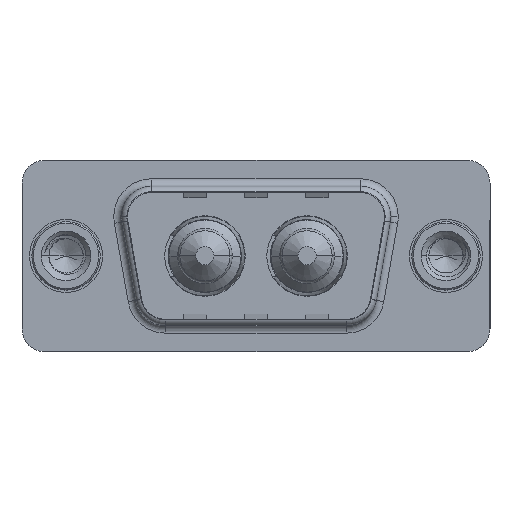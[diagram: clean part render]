
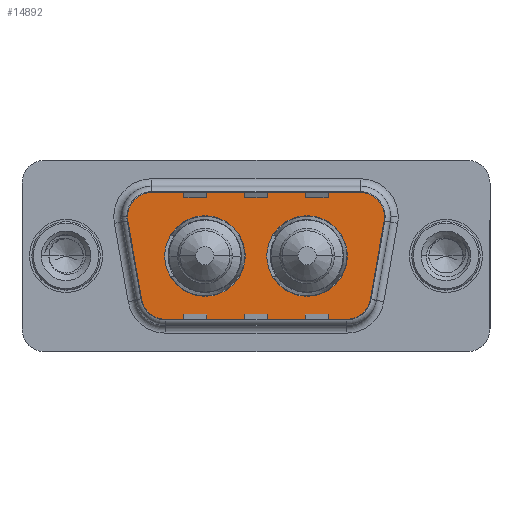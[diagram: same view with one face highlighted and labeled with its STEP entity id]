
A CAD part, top view. The second image highlights one B-rep face of the part: STEP entity #14892.
In plain terms, the highlighted planar face has unit normal (0, 0, 1).
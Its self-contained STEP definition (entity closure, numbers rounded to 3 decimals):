
#26 = CARTESIAN_POINT ( 'NONE',  ( 6.459, -4.9, 0. ) ) ;
#253 = ORIENTED_EDGE ( 'NONE', *, *, #2619, .T. ) ;
#300 = VERTEX_POINT ( 'NONE', #6458 ) ;
#446 = ORIENTED_EDGE ( 'NONE', *, *, #7942, .T. ) ;
#957 = LINE ( 'NONE', #13307, #3963 ) ;
#961 = CARTESIAN_POINT ( 'NONE',  ( 6.459, -2.9, 0. ) ) ;
#1237 = CARTESIAN_POINT ( 'NONE',  ( 15.86, 0., 0. ) ) ;
#1361 = CIRCLE ( 'NONE', #2441, 2. ) ;
#1375 = VERTEX_POINT ( 'NONE', #12462 ) ;
#1765 = ORIENTED_EDGE ( 'NONE', *, *, #13793, .F. ) ;
#1988 = VERTEX_POINT ( 'NONE', #5027 ) ;
#2060 = DIRECTION ( 'NONE',  ( -1., 0., 0. ) ) ;
#2064 = ORIENTED_EDGE ( 'NONE', *, *, #10052, .F. ) ;
#2158 = DIRECTION ( 'NONE',  ( 1., 0., 0. ) ) ;
#2235 = VERTEX_POINT ( 'NONE', #4317 ) ;
#2344 = DIRECTION ( 'NONE',  ( 1., 0., 0. ) ) ;
#2354 = CARTESIAN_POINT ( 'NONE',  ( 15.86, 0., 0. ) ) ;
#2430 = AXIS2_PLACEMENT_3D ( 'NONE', #9851, #2757, #10985 ) ;
#2441 = AXIS2_PLACEMENT_3D ( 'NONE', #10325, #7790, #4659 ) ;
#2619 = EDGE_CURVE ( 'NONE', #10789, #7506, #4810, .T. ) ;
#2757 = DIRECTION ( 'NONE',  ( 0., 0., 1. ) ) ;
#2855 = EDGE_LOOP ( 'NONE', ( #10129, #11180, #253, #5658, #10175, #11363, #446, #11546, #11727 ) ) ;
#3090 = DIRECTION ( 'NONE',  ( 0., 0., 1. ) ) ;
#3449 = CARTESIAN_POINT ( 'NONE',  ( 5.436, 4.9, 0. ) ) ;
#3522 = DIRECTION ( 'NONE',  ( 1., 0., 0. ) ) ;
#3548 = CARTESIAN_POINT ( 'NONE',  ( 6.49, 0., 0. ) ) ;
#3632 = CIRCLE ( 'NONE', #7813, 2.65 ) ;
#3662 = CARTESIAN_POINT ( 'NONE',  ( 21.564, 2.9, 0. ) ) ;
#3733 = EDGE_CURVE ( 'NONE', #7506, #4119, #11805, .T. ) ;
#3963 = VECTOR ( 'NONE', #10997, 1000. ) ;
#4089 = VECTOR ( 'NONE', #13083, 1000. ) ;
#4119 = VERTEX_POINT ( 'NONE', #11343 ) ;
#4190 = VERTEX_POINT ( 'NONE', #13928 ) ;
#4317 = CARTESIAN_POINT ( 'NONE',  ( 6.459, -4.9, 0. ) ) ;
#4391 = DIRECTION ( 'NONE',  ( -1., 0., 0. ) ) ;
#4404 = CARTESIAN_POINT ( 'NONE',  ( 13.21, 0., 0. ) ) ;
#4413 = DIRECTION ( 'NONE',  ( -1., 0., 0. ) ) ;
#4659 = DIRECTION ( 'NONE',  ( 1., 0., 0. ) ) ;
#4764 = FACE_OUTER_BOUND ( 'NONE', #2855, .T. ) ;
#4810 = CIRCLE ( 'NONE', #6948, 2. ) ;
#4905 = CIRCLE ( 'NONE', #13052, 2. ) ;
#5022 = EDGE_CURVE ( 'NONE', #6869, #5392, #1361, .T. ) ;
#5027 = CARTESIAN_POINT ( 'NONE',  ( 20.511, -3.247, 0. ) ) ;
#5128 = CARTESIAN_POINT ( 'NONE',  ( 9.14, 0., 0. ) ) ;
#5231 = EDGE_LOOP ( 'NONE', ( #13299, #6160 ) ) ;
#5392 = VERTEX_POINT ( 'NONE', #10147 ) ;
#5588 = AXIS2_PLACEMENT_3D ( 'NONE', #1237, #9449, #2344 ) ;
#5658 = ORIENTED_EDGE ( 'NONE', *, *, #3733, .T. ) ;
#5744 = DIRECTION ( 'NONE',  ( 0., 0., 1. ) ) ;
#5909 = FACE_BOUND ( 'NONE', #5231, .T. ) ;
#5912 = VERTEX_POINT ( 'NONE', #4404 ) ;
#6074 = CARTESIAN_POINT ( 'NONE',  ( 21.534, 2.553, 0. ) ) ;
#6160 = ORIENTED_EDGE ( 'NONE', *, *, #6797, .F. ) ;
#6341 = EDGE_CURVE ( 'NONE', #1375, #2235, #4905, .T. ) ;
#6362 = DIRECTION ( 'NONE',  ( 1., 0., 0. ) ) ;
#6458 = CARTESIAN_POINT ( 'NONE',  ( 18.51, 0., 0. ) ) ;
#6551 = DIRECTION ( 'NONE',  ( 0., 0., 1. ) ) ;
#6797 = EDGE_CURVE ( 'NONE', #12501, #10873, #3632, .T. ) ;
#6869 = VERTEX_POINT ( 'NONE', #7654 ) ;
#6948 = AXIS2_PLACEMENT_3D ( 'NONE', #14249, #10510, #4391 ) ;
#7095 = EDGE_CURVE ( 'NONE', #4190, #1988, #12080, .T. ) ;
#7120 = EDGE_LOOP ( 'NONE', ( #2064, #1765 ) ) ;
#7262 = LINE ( 'NONE', #6074, #4089 ) ;
#7303 = EDGE_CURVE ( 'NONE', #2235, #4190, #7529, .T. ) ;
#7351 = AXIS2_PLACEMENT_3D ( 'NONE', #2354, #10627, #3522 ) ;
#7506 = VERTEX_POINT ( 'NONE', #3662 ) ;
#7529 = LINE ( 'NONE', #26, #12984 ) ;
#7654 = CARTESIAN_POINT ( 'NONE',  ( 5.436, 4.9, 0. ) ) ;
#7694 = CARTESIAN_POINT ( 'NONE',  ( 18.541, -2.9, 0. ) ) ;
#7790 = DIRECTION ( 'NONE',  ( 0., 0., 1. ) ) ;
#7813 = AXIS2_PLACEMENT_3D ( 'NONE', #5128, #13360, #6362 ) ;
#7942 = EDGE_CURVE ( 'NONE', #5392, #1375, #957, .T. ) ;
#8224 = CARTESIAN_POINT ( 'NONE',  ( 19.564, 2.9, 0. ) ) ;
#9158 = DIRECTION ( 'NONE',  ( 0., 0., 1. ) ) ;
#9449 = DIRECTION ( 'NONE',  ( 0., 0., 1. ) ) ;
#9851 = CARTESIAN_POINT ( 'NONE',  ( 9.14, 0., 0. ) ) ;
#10033 = AXIS2_PLACEMENT_3D ( 'NONE', #7694, #6551, #14744 ) ;
#10052 = EDGE_CURVE ( 'NONE', #300, #5912, #10316, .T. ) ;
#10123 = CIRCLE ( 'NONE', #2430, 2.65 ) ;
#10129 = ORIENTED_EDGE ( 'NONE', *, *, #7095, .T. ) ;
#10147 = CARTESIAN_POINT ( 'NONE',  ( 3.466, 2.553, 0. ) ) ;
#10175 = ORIENTED_EDGE ( 'NONE', *, *, #12455, .T. ) ;
#10192 = CARTESIAN_POINT ( 'NONE',  ( 18.541, -2.9, 0. ) ) ;
#10316 = CIRCLE ( 'NONE', #7351, 2.65 ) ;
#10325 = CARTESIAN_POINT ( 'NONE',  ( 5.436, 2.9, 0. ) ) ;
#10510 = DIRECTION ( 'NONE',  ( 0., 0., 1. ) ) ;
#10605 = DIRECTION ( 'NONE',  ( -1., 0., 0. ) ) ;
#10627 = DIRECTION ( 'NONE',  ( 0., 0., 1. ) ) ;
#10676 = AXIS2_PLACEMENT_3D ( 'NONE', #10192, #3090, #11315 ) ;
#10735 = FACE_BOUND ( 'NONE', #7120, .T. ) ;
#10755 = CIRCLE ( 'NONE', #5588, 2.65 ) ;
#10789 = VERTEX_POINT ( 'NONE', #14126 ) ;
#10843 = CARTESIAN_POINT ( 'NONE',  ( 11.79, 0., 0. ) ) ;
#10873 = VERTEX_POINT ( 'NONE', #10843 ) ;
#10985 = DIRECTION ( 'NONE',  ( 1., 0., 0. ) ) ;
#10997 = DIRECTION ( 'NONE',  ( 0.174, -0.985, 0. ) ) ;
#11180 = ORIENTED_EDGE ( 'NONE', *, *, #12607, .T. ) ;
#11315 = DIRECTION ( 'NONE',  ( 1., 0., 0. ) ) ;
#11343 = CARTESIAN_POINT ( 'NONE',  ( 19.564, 4.9, 0. ) ) ;
#11363 = ORIENTED_EDGE ( 'NONE', *, *, #5022, .T. ) ;
#11540 = EDGE_CURVE ( 'NONE', #10873, #12501, #10123, .T. ) ;
#11546 = ORIENTED_EDGE ( 'NONE', *, *, #6341, .T. ) ;
#11727 = ORIENTED_EDGE ( 'NONE', *, *, #7303, .T. ) ;
#11805 = CIRCLE ( 'NONE', #12057, 2. ) ;
#11833 = LINE ( 'NONE', #3449, #14960 ) ;
#12057 = AXIS2_PLACEMENT_3D ( 'NONE', #8224, #5744, #4413 ) ;
#12080 = CIRCLE ( 'NONE', #10676, 2. ) ;
#12455 = EDGE_CURVE ( 'NONE', #4119, #6869, #11833, .T. ) ;
#12462 = CARTESIAN_POINT ( 'NONE',  ( 4.489, -3.247, 0. ) ) ;
#12501 = VERTEX_POINT ( 'NONE', #3548 ) ;
#12607 = EDGE_CURVE ( 'NONE', #1988, #10789, #7262, .T. ) ;
#12984 = VECTOR ( 'NONE', #2158, 1000. ) ;
#13052 = AXIS2_PLACEMENT_3D ( 'NONE', #961, #9158, #2060 ) ;
#13083 = DIRECTION ( 'NONE',  ( 0.174, 0.985, 0. ) ) ;
#13299 = ORIENTED_EDGE ( 'NONE', *, *, #11540, .F. ) ;
#13307 = CARTESIAN_POINT ( 'NONE',  ( 3.466, 2.553, 0. ) ) ;
#13360 = DIRECTION ( 'NONE',  ( 0., 0., 1. ) ) ;
#13548 = PLANE ( 'NONE',  #10033 ) ;
#13793 = EDGE_CURVE ( 'NONE', #5912, #300, #10755, .T. ) ;
#13928 = CARTESIAN_POINT ( 'NONE',  ( 18.541, -4.9, 0. ) ) ;
#14126 = CARTESIAN_POINT ( 'NONE',  ( 21.534, 2.553, 0. ) ) ;
#14249 = CARTESIAN_POINT ( 'NONE',  ( 19.564, 2.9, 0. ) ) ;
#14744 = DIRECTION ( 'NONE',  ( 1., 0., 0. ) ) ;
#14892 = ADVANCED_FACE ( 'NONE', ( #10735, #5909, #4764 ), #13548, .T. ) ;
#14960 = VECTOR ( 'NONE', #10605, 1000. ) ;
